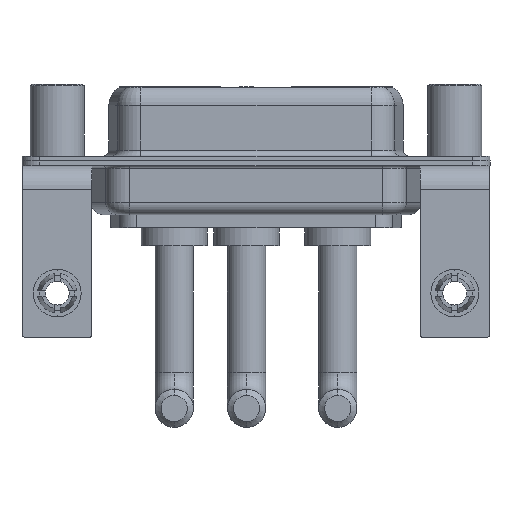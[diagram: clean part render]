
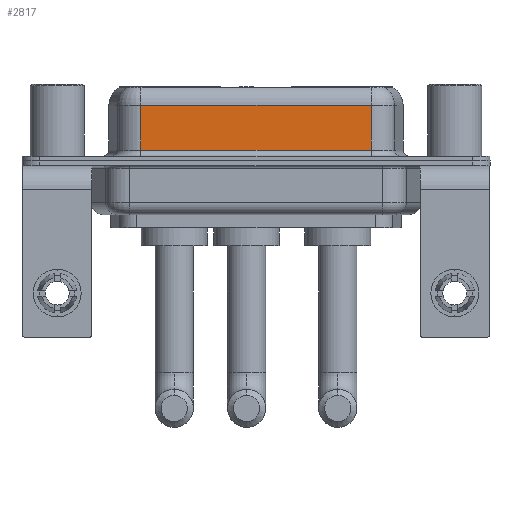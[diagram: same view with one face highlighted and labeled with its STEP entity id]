
A CAD part, front view. The second image highlights one B-rep face of the part: STEP entity #2817.
In plain terms, the highlighted planar face has unit normal (0, -1, 0).
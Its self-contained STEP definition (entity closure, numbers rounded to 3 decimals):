
#333 = EDGE_CURVE ( 'NONE', #17252, #11236, #16276, .T. ) ;
#723 = DIRECTION ( 'NONE',  ( 0., 0., 1. ) ) ;
#1033 = VECTOR ( 'NONE', #8488, 1000. ) ;
#1594 = DIRECTION ( 'NONE',  ( -1., 0., 0. ) ) ;
#1971 = FACE_OUTER_BOUND ( 'NONE', #3259, .T. ) ;
#2817 = ADVANCED_FACE ( 'NONE', ( #1971 ), #7154, .F. ) ;
#2853 = AXIS2_PLACEMENT_3D ( 'NONE', #4432, #16599, #723 ) ;
#2934 = LINE ( 'NONE', #8266, #13654 ) ;
#3068 = CARTESIAN_POINT ( 'NONE',  ( 26.287, -3.95, 6.4 ) ) ;
#3259 = EDGE_LOOP ( 'NONE', ( #13901, #14987, #7479, #5387 ) ) ;
#4206 = DIRECTION ( 'NONE',  ( 0., 0., -1. ) ) ;
#4432 = CARTESIAN_POINT ( 'NONE',  ( 26.287, -3.95, 6.4 ) ) ;
#4539 = VECTOR ( 'NONE', #10987, 1000. ) ;
#4804 = CARTESIAN_POINT ( 'NONE',  ( 26.287, -3.95, 0.9 ) ) ;
#5308 = VECTOR ( 'NONE', #4206, 1000. ) ;
#5387 = ORIENTED_EDGE ( 'NONE', *, *, #11066, .T. ) ;
#6933 = EDGE_CURVE ( 'NONE', #17252, #11039, #2934, .T. ) ;
#7154 = PLANE ( 'NONE',  #2853 ) ;
#7172 = LINE ( 'NONE', #15048, #1033 ) ;
#7479 = ORIENTED_EDGE ( 'NONE', *, *, #17050, .T. ) ;
#8266 = CARTESIAN_POINT ( 'NONE',  ( 26.287, -3.95, 4.65 ) ) ;
#8488 = DIRECTION ( 'NONE',  ( 1., 0., 0. ) ) ;
#8641 = CARTESIAN_POINT ( 'NONE',  ( 7.013, -3.95, 0.9 ) ) ;
#10987 = DIRECTION ( 'NONE',  ( 0., 0., -1. ) ) ;
#11039 = VERTEX_POINT ( 'NONE', #13827 ) ;
#11066 = EDGE_CURVE ( 'NONE', #16722, #11236, #7172, .T. ) ;
#11072 = CARTESIAN_POINT ( 'NONE',  ( 26.287, -3.95, 4.65 ) ) ;
#11236 = VERTEX_POINT ( 'NONE', #4804 ) ;
#13457 = CARTESIAN_POINT ( 'NONE',  ( 7.013, -3.95, 6.4 ) ) ;
#13654 = VECTOR ( 'NONE', #1594, 1000. ) ;
#13827 = CARTESIAN_POINT ( 'NONE',  ( 7.013, -3.95, 4.65 ) ) ;
#13901 = ORIENTED_EDGE ( 'NONE', *, *, #333, .F. ) ;
#14987 = ORIENTED_EDGE ( 'NONE', *, *, #6933, .T. ) ;
#15048 = CARTESIAN_POINT ( 'NONE',  ( 26.287, -3.95, 0.9 ) ) ;
#16153 = LINE ( 'NONE', #13457, #4539 ) ;
#16276 = LINE ( 'NONE', #3068, #5308 ) ;
#16599 = DIRECTION ( 'NONE',  ( 0., 1., 0. ) ) ;
#16722 = VERTEX_POINT ( 'NONE', #8641 ) ;
#17050 = EDGE_CURVE ( 'NONE', #11039, #16722, #16153, .T. ) ;
#17252 = VERTEX_POINT ( 'NONE', #11072 ) ;
